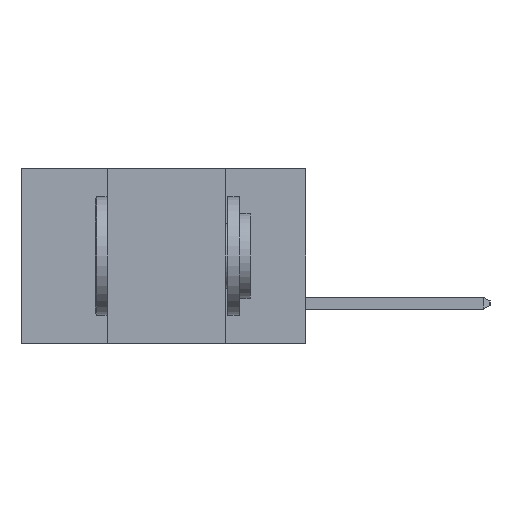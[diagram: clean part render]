
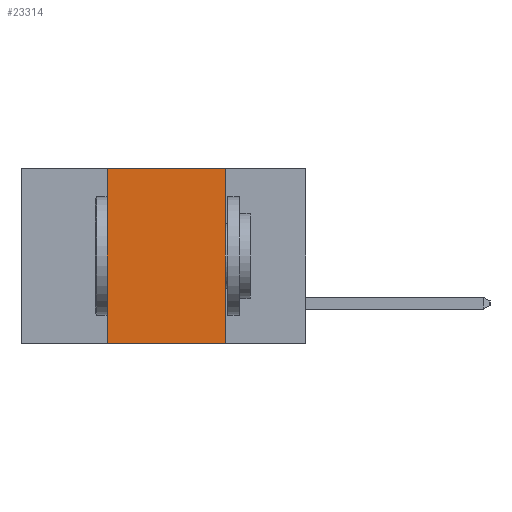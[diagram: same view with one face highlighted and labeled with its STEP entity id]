
A CAD part, left-side view. The second image highlights one B-rep face of the part: STEP entity #23314.
In plain terms, the highlighted planar face has unit normal (-1, 0, 0).
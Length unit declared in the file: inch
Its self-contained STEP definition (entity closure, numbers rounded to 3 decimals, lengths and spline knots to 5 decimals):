
#775 = ORIENTED_EDGE ( 'NONE', *, *, #12142, .F. ) ;
#977 = EDGE_CURVE ( 'NONE', #15836, #7664, #23592, .T. ) ;
#1216 = CARTESIAN_POINT ( 'NONE',  ( 0., 0.17, 0. ) ) ;
#2243 = LINE ( 'NONE', #16414, #6140 ) ;
#2906 = VERTEX_POINT ( 'NONE', #11014 ) ;
#3159 = DIRECTION ( 'NONE',  ( 0., 0., -1. ) ) ;
#3243 = CARTESIAN_POINT ( 'NONE',  ( 0., 0.17, 0. ) ) ;
#3922 = VECTOR ( 'NONE', #18727, 39.37008 ) ;
#6140 = VECTOR ( 'NONE', #20201, 39.37008 ) ;
#6902 = CARTESIAN_POINT ( 'NONE',  ( 0., 0.42, -0.37 ) ) ;
#7664 = VERTEX_POINT ( 'NONE', #3243 ) ;
#8818 = DIRECTION ( 'NONE',  ( 1., 0., 0. ) ) ;
#9117 = LINE ( 'NONE', #21595, #13541 ) ;
#10169 = VERTEX_POINT ( 'NONE', #6902 ) ;
#10407 = ORIENTED_EDGE ( 'NONE', *, *, #22642, .F. ) ;
#10622 = CARTESIAN_POINT ( 'NONE',  ( 0., 0.6, 0. ) ) ;
#11014 = CARTESIAN_POINT ( 'NONE',  ( 0., 0.17, -0.37 ) ) ;
#12142 = EDGE_CURVE ( 'NONE', #7664, #2906, #24136, .T. ) ;
#12481 = DIRECTION ( 'NONE',  ( 0., -1., 0. ) ) ;
#13541 = VECTOR ( 'NONE', #12481, 39.37008 ) ;
#15765 = CARTESIAN_POINT ( 'NONE',  ( 0., 0.6, 0. ) ) ;
#15836 = VERTEX_POINT ( 'NONE', #17439 ) ;
#16414 = CARTESIAN_POINT ( 'NONE',  ( 0., 0.42, 0. ) ) ;
#16661 = ORIENTED_EDGE ( 'NONE', *, *, #977, .F. ) ;
#16942 = ORIENTED_EDGE ( 'NONE', *, *, #24381, .T. ) ;
#17439 = CARTESIAN_POINT ( 'NONE',  ( 0., 0.42, 0. ) ) ;
#18319 = PLANE ( 'NONE',  #22557 ) ;
#18727 = DIRECTION ( 'NONE',  ( 0., -1., 0. ) ) ;
#20201 = DIRECTION ( 'NONE',  ( 0., 0., 1. ) ) ;
#21595 = CARTESIAN_POINT ( 'NONE',  ( 0., 0.6, -0.37 ) ) ;
#22141 = DIRECTION ( 'NONE',  ( 0., 0., -1. ) ) ;
#22557 = AXIS2_PLACEMENT_3D ( 'NONE', #10622, #8818, #22141 ) ;
#22642 = EDGE_CURVE ( 'NONE', #10169, #15836, #2243, .T. ) ;
#22664 = EDGE_LOOP ( 'NONE', ( #775, #16661, #10407, #16942 ) ) ;
#23314 = ADVANCED_FACE ( 'NONE', ( #24237 ), #18319, .F. ) ;
#23560 = VECTOR ( 'NONE', #3159, 39.37008 ) ;
#23592 = LINE ( 'NONE', #15765, #3922 ) ;
#24136 = LINE ( 'NONE', #1216, #23560 ) ;
#24237 = FACE_OUTER_BOUND ( 'NONE', #22664, .T. ) ;
#24381 = EDGE_CURVE ( 'NONE', #10169, #2906, #9117, .T. ) ;
